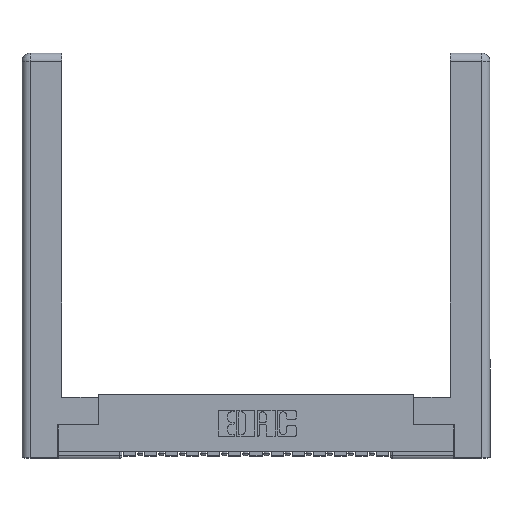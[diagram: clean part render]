
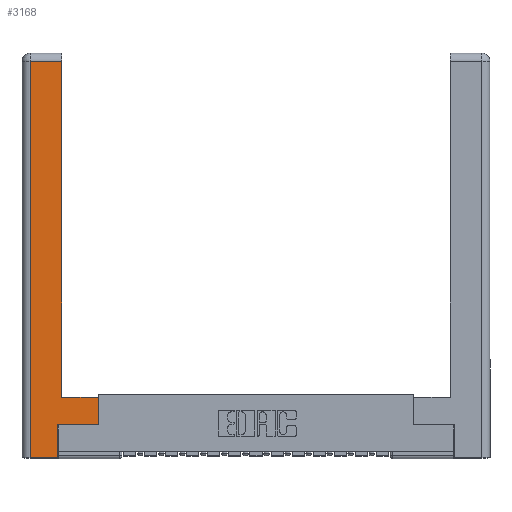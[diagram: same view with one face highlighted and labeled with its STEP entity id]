
A CAD part, top view. The second image highlights one B-rep face of the part: STEP entity #3168.
In plain terms, the highlighted planar face has unit normal (0, 0, 1).
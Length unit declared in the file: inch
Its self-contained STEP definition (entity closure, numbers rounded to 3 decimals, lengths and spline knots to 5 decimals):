
#292 = DIRECTION ( 'NONE',  ( 1., 0., 0. ) ) ;
#876 = ORIENTED_EDGE ( 'NONE', *, *, #18062, .T. ) ;
#928 = DIRECTION ( 'NONE',  ( 0., -1., 0. ) ) ;
#967 = CARTESIAN_POINT ( 'NONE',  ( 0.295, 0.45, 0. ) ) ;
#1000 = EDGE_CURVE ( 'NONE', #6456, #18020, #18007, .T. ) ;
#1183 = DIRECTION ( 'NONE',  ( 0., 1., 0. ) ) ;
#1248 = VERTEX_POINT ( 'NONE', #7182 ) ;
#1526 = VECTOR ( 'NONE', #292, 39.37008 ) ;
#1543 = CARTESIAN_POINT ( 'NONE',  ( 0.565, 0.245, 0. ) ) ;
#1647 = VECTOR ( 'NONE', #928, 39.37008 ) ;
#1770 = LINE ( 'NONE', #12980, #1526 ) ;
#2142 = AXIS2_PLACEMENT_3D ( 'NONE', #4075, #2496, #8162 ) ;
#2289 = CARTESIAN_POINT ( 'NONE',  ( 0.565, 0.45, 0. ) ) ;
#2496 = DIRECTION ( 'NONE',  ( 0., 0., -1. ) ) ;
#2780 = CARTESIAN_POINT ( 'NONE',  ( 0.0615, 0., 0. ) ) ;
#2933 = VECTOR ( 'NONE', #1183, 39.37008 ) ;
#3168 = ADVANCED_FACE ( 'NONE', ( #16769 ), #15184, .F. ) ;
#3995 = CARTESIAN_POINT ( 'NONE',  ( 0.265, 0.245, 0. ) ) ;
#4075 = CARTESIAN_POINT ( 'NONE',  ( 0., 0., 0. ) ) ;
#4191 = EDGE_CURVE ( 'NONE', #15111, #11196, #18052, .T. ) ;
#4287 = LINE ( 'NONE', #9680, #11952 ) ;
#4415 = ORIENTED_EDGE ( 'NONE', *, *, #16503, .T. ) ;
#4480 = DIRECTION ( 'NONE',  ( 1., 0., 0. ) ) ;
#4564 = CARTESIAN_POINT ( 'NONE',  ( 0.565, 0.45, 0. ) ) ;
#4788 = VECTOR ( 'NONE', #4480, 39.37008 ) ;
#5383 = LINE ( 'NONE', #3995, #17524 ) ;
#6338 = CARTESIAN_POINT ( 'NONE',  ( 0.295, 0.45, 0. ) ) ;
#6392 = CARTESIAN_POINT ( 'NONE',  ( 0.0615, 0., 0. ) ) ;
#6456 = VERTEX_POINT ( 'NONE', #967 ) ;
#6611 = LINE ( 'NONE', #6338, #14230 ) ;
#7042 = VERTEX_POINT ( 'NONE', #2780 ) ;
#7182 = CARTESIAN_POINT ( 'NONE',  ( 0.265, 0., 0. ) ) ;
#7273 = ORIENTED_EDGE ( 'NONE', *, *, #13899, .T. ) ;
#8162 = DIRECTION ( 'NONE',  ( -1., 0., 0. ) ) ;
#8307 = ORIENTED_EDGE ( 'NONE', *, *, #1000, .T. ) ;
#8640 = LINE ( 'NONE', #17167, #4788 ) ;
#9144 = VERTEX_POINT ( 'NONE', #13638 ) ;
#9314 = EDGE_CURVE ( 'NONE', #9144, #15111, #1770, .T. ) ;
#9665 = DIRECTION ( 'NONE',  ( 0., 1., 0. ) ) ;
#9680 = CARTESIAN_POINT ( 'NONE',  ( 0.0615, 2.94, 0. ) ) ;
#10254 = EDGE_LOOP ( 'NONE', ( #8307, #4415, #876, #11300, #10736, #13545, #17716, #7273 ) ) ;
#10736 = ORIENTED_EDGE ( 'NONE', *, *, #14553, .T. ) ;
#11196 = VERTEX_POINT ( 'NONE', #4564 ) ;
#11300 = ORIENTED_EDGE ( 'NONE', *, *, #14251, .T. ) ;
#11351 = DIRECTION ( 'NONE',  ( -1., 0., 0. ) ) ;
#11952 = VECTOR ( 'NONE', #11351, 39.37008 ) ;
#12459 = DIRECTION ( 'NONE',  ( 0., 1., 0. ) ) ;
#12980 = CARTESIAN_POINT ( 'NONE',  ( 0.565, 0.245, 0. ) ) ;
#13545 = ORIENTED_EDGE ( 'NONE', *, *, #9314, .T. ) ;
#13638 = CARTESIAN_POINT ( 'NONE',  ( 0.265, 0.245, 0. ) ) ;
#13644 = CARTESIAN_POINT ( 'NONE',  ( 0.295, 3., 0. ) ) ;
#13899 = EDGE_CURVE ( 'NONE', #11196, #6456, #6611, .T. ) ;
#14230 = VECTOR ( 'NONE', #14839, 39.37008 ) ;
#14251 = EDGE_CURVE ( 'NONE', #7042, #1248, #8640, .T. ) ;
#14553 = EDGE_CURVE ( 'NONE', #1248, #9144, #5383, .T. ) ;
#14678 = CARTESIAN_POINT ( 'NONE',  ( 0.0615, 2.94, 0. ) ) ;
#14839 = DIRECTION ( 'NONE',  ( -1., 0., 0. ) ) ;
#15111 = VERTEX_POINT ( 'NONE', #1543 ) ;
#15184 = PLANE ( 'NONE',  #2142 ) ;
#16487 = VECTOR ( 'NONE', #12459, 39.37008 ) ;
#16503 = EDGE_CURVE ( 'NONE', #18020, #17080, #4287, .T. ) ;
#16769 = FACE_OUTER_BOUND ( 'NONE', #10254, .T. ) ;
#17080 = VERTEX_POINT ( 'NONE', #14678 ) ;
#17167 = CARTESIAN_POINT ( 'NONE',  ( 0.265, 0., 0. ) ) ;
#17524 = VECTOR ( 'NONE', #9665, 39.37008 ) ;
#17699 = CARTESIAN_POINT ( 'NONE',  ( 0.295, 2.94, 0. ) ) ;
#17716 = ORIENTED_EDGE ( 'NONE', *, *, #4191, .T. ) ;
#17892 = LINE ( 'NONE', #6392, #1647 ) ;
#18007 = LINE ( 'NONE', #13644, #16487 ) ;
#18020 = VERTEX_POINT ( 'NONE', #17699 ) ;
#18052 = LINE ( 'NONE', #2289, #2933 ) ;
#18062 = EDGE_CURVE ( 'NONE', #17080, #7042, #17892, .T. ) ;
